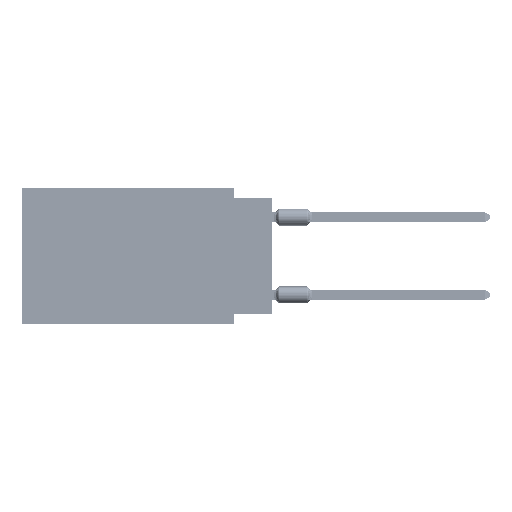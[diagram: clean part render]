
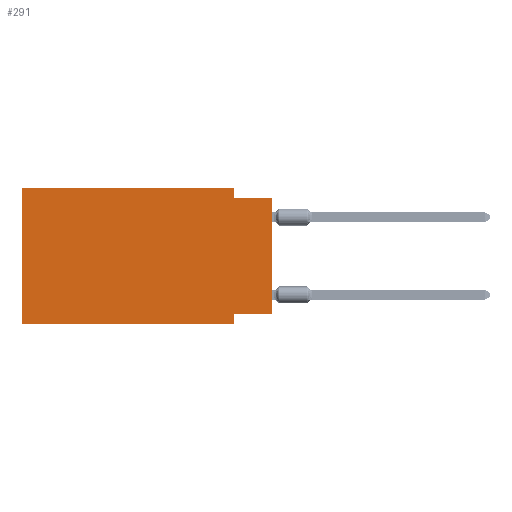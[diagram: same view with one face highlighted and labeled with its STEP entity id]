
A CAD part, left-side view. The second image highlights one B-rep face of the part: STEP entity #291.
In plain terms, the highlighted planar face has unit normal (-1, 0, 0).
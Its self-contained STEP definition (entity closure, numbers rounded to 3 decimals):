
#291 = ADVANCED_FACE ( 'NONE', ( #21633 ), #72158, .F. ) ;
#5909 = DIRECTION ( 'NONE',  ( 0., 0., -1. ) ) ;
#5969 = VECTOR ( 'NONE', #82166, 1000. ) ;
#6074 = DIRECTION ( 'NONE',  ( 0., 0., -1. ) ) ;
#6547 = ORIENTED_EDGE ( 'NONE', *, *, #9270, .T. ) ;
#9270 = EDGE_CURVE ( 'NONE', #107478, #55051, #13690, .T. ) ;
#10984 = VECTOR ( 'NONE', #6074, 1000. ) ;
#11124 = CARTESIAN_POINT ( 'NONE',  ( 0., 2.54, -0.635 ) ) ;
#12440 = EDGE_CURVE ( 'NONE', #107478, #104794, #70521, .T. ) ;
#13690 = LINE ( 'NONE', #47887, #5969 ) ;
#16508 = CARTESIAN_POINT ( 'NONE',  ( 0., 16.383, -8.89 ) ) ;
#18534 = VECTOR ( 'NONE', #59920, 1000. ) ;
#21633 = FACE_OUTER_BOUND ( 'NONE', #46931, .T. ) ;
#21786 = LINE ( 'NONE', #32410, #10984 ) ;
#24450 = VERTEX_POINT ( 'NONE', #71417 ) ;
#26849 = ORIENTED_EDGE ( 'NONE', *, *, #78373, .F. ) ;
#27070 = EDGE_CURVE ( 'NONE', #24450, #96929, #105320, .T. ) ;
#30016 = ORIENTED_EDGE ( 'NONE', *, *, #12440, .F. ) ;
#30793 = LINE ( 'NONE', #99834, #37517 ) ;
#31486 = VECTOR ( 'NONE', #52539, 1000. ) ;
#32145 = CARTESIAN_POINT ( 'NONE',  ( 0., 0., 0. ) ) ;
#32334 = VECTOR ( 'NONE', #58522, 1000. ) ;
#32410 = CARTESIAN_POINT ( 'NONE',  ( 0., 2.54, -8.89 ) ) ;
#37517 = VECTOR ( 'NONE', #99274, 1000. ) ;
#39403 = DIRECTION ( 'NONE',  ( 0., -1., 0. ) ) ;
#42550 = EDGE_CURVE ( 'NONE', #96929, #55051, #21786, .T. ) ;
#43508 = EDGE_CURVE ( 'NONE', #24450, #66420, #59636, .T. ) ;
#46931 = EDGE_LOOP ( 'NONE', ( #94204, #26849, #52269, #101340, #30016, #6547, #60617, #93589 ) ) ;
#47887 = CARTESIAN_POINT ( 'NONE',  ( 0., 16.383, -8.89 ) ) ;
#48288 = LINE ( 'NONE', #97722, #86698 ) ;
#52269 = ORIENTED_EDGE ( 'NONE', *, *, #88830, .F. ) ;
#52539 = DIRECTION ( 'NONE',  ( 0., 0., 1. ) ) ;
#55051 = VERTEX_POINT ( 'NONE', #62888 ) ;
#58135 = CARTESIAN_POINT ( 'NONE',  ( 0., 2.54, 0. ) ) ;
#58522 = DIRECTION ( 'NONE',  ( 0., 0., 1. ) ) ;
#59636 = LINE ( 'NONE', #32145, #32334 ) ;
#59920 = DIRECTION ( 'NONE',  ( 0., 1., 0. ) ) ;
#60617 = ORIENTED_EDGE ( 'NONE', *, *, #42550, .F. ) ;
#62888 = CARTESIAN_POINT ( 'NONE',  ( 0., 2.54, -8.89 ) ) ;
#66420 = VERTEX_POINT ( 'NONE', #104063 ) ;
#70289 = AXIS2_PLACEMENT_3D ( 'NONE', #82803, #89574, #5909 ) ;
#70521 = LINE ( 'NONE', #102529, #31486 ) ;
#71417 = CARTESIAN_POINT ( 'NONE',  ( 0., 0., -8.255 ) ) ;
#72158 = PLANE ( 'NONE',  #70289 ) ;
#78373 = EDGE_CURVE ( 'NONE', #99932, #66420, #30793, .T. ) ;
#78708 = VECTOR ( 'NONE', #39403, 1000. ) ;
#81529 = CARTESIAN_POINT ( 'NONE',  ( 0., 16.383, 0. ) ) ;
#82166 = DIRECTION ( 'NONE',  ( 0., -1., 0. ) ) ;
#82803 = CARTESIAN_POINT ( 'NONE',  ( 0., 16.383, 0. ) ) ;
#86698 = VECTOR ( 'NONE', #108342, 1000. ) ;
#87213 = LINE ( 'NONE', #81529, #78708 ) ;
#87411 = CARTESIAN_POINT ( 'NONE',  ( 0., 0., -8.255 ) ) ;
#88830 = EDGE_CURVE ( 'NONE', #92773, #99932, #48288, .T. ) ;
#89574 = DIRECTION ( 'NONE',  ( 1., 0., 0. ) ) ;
#92773 = VERTEX_POINT ( 'NONE', #58135 ) ;
#93589 = ORIENTED_EDGE ( 'NONE', *, *, #27070, .F. ) ;
#94204 = ORIENTED_EDGE ( 'NONE', *, *, #43508, .T. ) ;
#95902 = CARTESIAN_POINT ( 'NONE',  ( 0., 16.383, 0. ) ) ;
#96929 = VERTEX_POINT ( 'NONE', #107859 ) ;
#97722 = CARTESIAN_POINT ( 'NONE',  ( 0., 2.54, 0. ) ) ;
#99274 = DIRECTION ( 'NONE',  ( 0., -1., 0. ) ) ;
#99834 = CARTESIAN_POINT ( 'NONE',  ( 0., 0., -0.635 ) ) ;
#99932 = VERTEX_POINT ( 'NONE', #11124 ) ;
#101340 = ORIENTED_EDGE ( 'NONE', *, *, #110022, .F. ) ;
#102529 = CARTESIAN_POINT ( 'NONE',  ( 0., 16.383, 0. ) ) ;
#104063 = CARTESIAN_POINT ( 'NONE',  ( 0., 0., -0.635 ) ) ;
#104794 = VERTEX_POINT ( 'NONE', #95902 ) ;
#105320 = LINE ( 'NONE', #87411, #18534 ) ;
#107478 = VERTEX_POINT ( 'NONE', #16508 ) ;
#107859 = CARTESIAN_POINT ( 'NONE',  ( 0., 2.54, -8.255 ) ) ;
#108342 = DIRECTION ( 'NONE',  ( 0., 0., -1. ) ) ;
#110022 = EDGE_CURVE ( 'NONE', #104794, #92773, #87213, .T. ) ;
